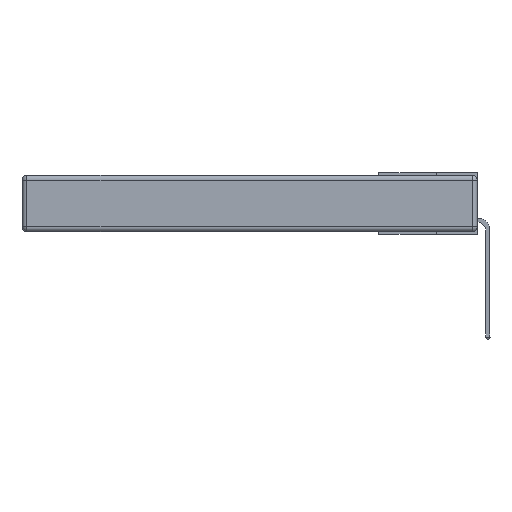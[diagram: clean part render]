
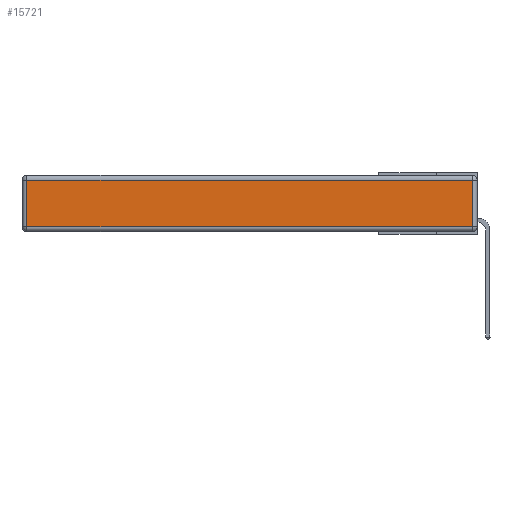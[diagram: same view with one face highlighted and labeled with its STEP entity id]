
A CAD part, left-side view. The second image highlights one B-rep face of the part: STEP entity #15721.
In plain terms, the highlighted planar face has unit normal (-1, 0, 0).
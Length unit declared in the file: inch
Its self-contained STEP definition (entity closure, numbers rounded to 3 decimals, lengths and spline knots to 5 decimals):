
#257 = VECTOR ( 'NONE', #10043, 39.37008 ) ;
#930 = EDGE_CURVE ( 'NONE', #18314, #10770, #8857, .T. ) ;
#1213 = EDGE_LOOP ( 'NONE', ( #4699, #19353, #7260, #16245 ) ) ;
#1668 = DIRECTION ( 'NONE',  ( -1., 0., 0. ) ) ;
#1686 = CARTESIAN_POINT ( 'NONE',  ( 0., 2.75, -0.03 ) ) ;
#2022 = LINE ( 'NONE', #4820, #14909 ) ;
#2746 = VECTOR ( 'NONE', #14867, 39.37008 ) ;
#3023 = CARTESIAN_POINT ( 'NONE',  ( 0., 0.03, -0.313 ) ) ;
#3026 = CARTESIAN_POINT ( 'NONE',  ( 0., 0., -0.313 ) ) ;
#3400 = CARTESIAN_POINT ( 'NONE',  ( 0., 2.72, -0.03 ) ) ;
#4372 = VECTOR ( 'NONE', #6121, 39.37008 ) ;
#4699 = ORIENTED_EDGE ( 'NONE', *, *, #930, .T. ) ;
#4820 = CARTESIAN_POINT ( 'NONE',  ( 0., 0.03, -0.343 ) ) ;
#4851 = VERTEX_POINT ( 'NONE', #19491 ) ;
#5400 = EDGE_CURVE ( 'NONE', #12642, #18314, #18576, .T. ) ;
#6121 = DIRECTION ( 'NONE',  ( 0., 0., -1. ) ) ;
#7027 = CARTESIAN_POINT ( 'NONE',  ( 0., 0., -0.343 ) ) ;
#7260 = ORIENTED_EDGE ( 'NONE', *, *, #19223, .T. ) ;
#8511 = CARTESIAN_POINT ( 'NONE',  ( 0., 2.72, -0.313 ) ) ;
#8857 = LINE ( 'NONE', #3026, #2746 ) ;
#9136 = AXIS2_PLACEMENT_3D ( 'NONE', #7027, #1668, #13450 ) ;
#9434 = CARTESIAN_POINT ( 'NONE',  ( 0., 2.72, -0.343 ) ) ;
#10043 = DIRECTION ( 'NONE',  ( 0., 1., 0. ) ) ;
#10770 = VERTEX_POINT ( 'NONE', #3023 ) ;
#12642 = VERTEX_POINT ( 'NONE', #3400 ) ;
#13450 = DIRECTION ( 'NONE',  ( 0., 0., 1. ) ) ;
#13651 = DIRECTION ( 'NONE',  ( 0., 0., 1. ) ) ;
#14867 = DIRECTION ( 'NONE',  ( 0., -1., 0. ) ) ;
#14909 = VECTOR ( 'NONE', #13651, 39.37008 ) ;
#15451 = FACE_OUTER_BOUND ( 'NONE', #1213, .T. ) ;
#15721 = ADVANCED_FACE ( 'NONE', ( #15451 ), #17029, .T. ) ;
#16245 = ORIENTED_EDGE ( 'NONE', *, *, #5400, .T. ) ;
#17029 = PLANE ( 'NONE',  #9136 ) ;
#17577 = LINE ( 'NONE', #1686, #257 ) ;
#18314 = VERTEX_POINT ( 'NONE', #8511 ) ;
#18576 = LINE ( 'NONE', #9434, #4372 ) ;
#19223 = EDGE_CURVE ( 'NONE', #4851, #12642, #17577, .T. ) ;
#19353 = ORIENTED_EDGE ( 'NONE', *, *, #20486, .T. ) ;
#19491 = CARTESIAN_POINT ( 'NONE',  ( 0., 0.03, -0.03 ) ) ;
#20486 = EDGE_CURVE ( 'NONE', #10770, #4851, #2022, .T. ) ;
